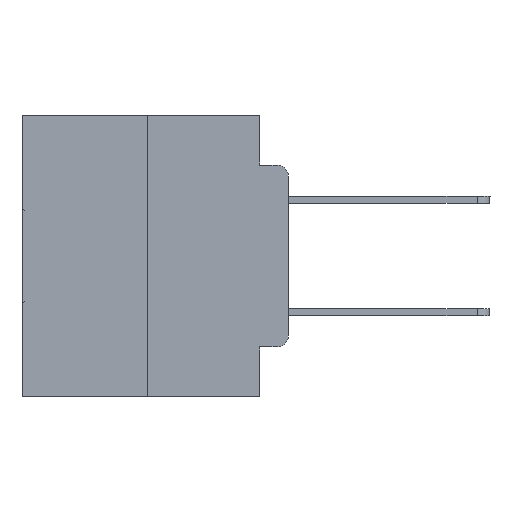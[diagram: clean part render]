
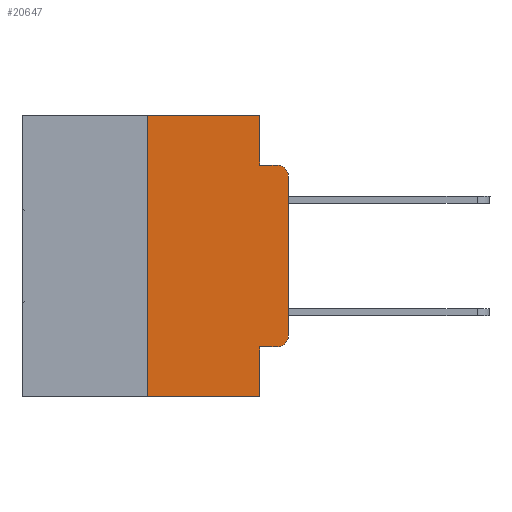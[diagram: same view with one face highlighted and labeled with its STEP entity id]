
A CAD part, left-side view. The second image highlights one B-rep face of the part: STEP entity #20647.
In plain terms, the highlighted planar face has unit normal (-1, 0, 0).
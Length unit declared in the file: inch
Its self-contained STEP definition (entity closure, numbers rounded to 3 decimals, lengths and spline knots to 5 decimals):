
#346 = CARTESIAN_POINT ( 'NONE',  ( 0., 0.051, 0. ) ) ;
#371 = DIRECTION ( 'NONE',  ( 0., 0., -1. ) ) ;
#406 = EDGE_CURVE ( 'NONE', #13097, #30478, #20807, .T. ) ;
#618 = VERTEX_POINT ( 'NONE', #19233 ) ;
#1803 = VERTEX_POINT ( 'NONE', #17296 ) ;
#1904 = EDGE_LOOP ( 'NONE', ( #2455, #10410, #29172, #29894, #11899, #6253, #25933, #15643, #28065, #16396 ) ) ;
#2161 = EDGE_CURVE ( 'NONE', #28129, #618, #17019, .T. ) ;
#2455 = ORIENTED_EDGE ( 'NONE', *, *, #9675, .T. ) ;
#3018 = FACE_OUTER_BOUND ( 'NONE', #1904, .T. ) ;
#3943 = LINE ( 'NONE', #21000, #8900 ) ;
#4062 = LINE ( 'NONE', #24683, #11263 ) ;
#4309 = VECTOR ( 'NONE', #19586, 39.37008 ) ;
#5219 = LINE ( 'NONE', #12419, #10873 ) ;
#5412 = EDGE_CURVE ( 'NONE', #27784, #13097, #4062, .T. ) ;
#5867 = DIRECTION ( 'NONE',  ( 1., 0., 0. ) ) ;
#6253 = ORIENTED_EDGE ( 'NONE', *, *, #5412, .F. ) ;
#6920 = DIRECTION ( 'NONE',  ( -1., 0., 0. ) ) ;
#7275 = EDGE_CURVE ( 'NONE', #27784, #618, #8908, .T. ) ;
#7495 = DIRECTION ( 'NONE',  ( 0., -1., 0. ) ) ;
#7608 = LINE ( 'NONE', #24013, #13200 ) ;
#8628 = DIRECTION ( 'NONE',  ( 0., -1., 0. ) ) ;
#8900 = VECTOR ( 'NONE', #16206, 39.37008 ) ;
#8908 = LINE ( 'NONE', #25203, #15261 ) ;
#9096 = VERTEX_POINT ( 'NONE', #24602 ) ;
#9675 = EDGE_CURVE ( 'NONE', #12359, #27761, #10745, .T. ) ;
#10410 = ORIENTED_EDGE ( 'NONE', *, *, #27595, .T. ) ;
#10500 = DIRECTION ( 'NONE',  ( 0., 0., 1. ) ) ;
#10649 = VECTOR ( 'NONE', #14969, 39.37008 ) ;
#10745 = LINE ( 'NONE', #26467, #4309 ) ;
#10873 = VECTOR ( 'NONE', #371, 39.37008 ) ;
#11010 = DIRECTION ( 'NONE',  ( 0., -1., 0. ) ) ;
#11263 = VECTOR ( 'NONE', #10500, 39.37008 ) ;
#11899 = ORIENTED_EDGE ( 'NONE', *, *, #406, .F. ) ;
#11920 = CARTESIAN_POINT ( 'NONE',  ( 0., 0.051, 0. ) ) ;
#12359 = VERTEX_POINT ( 'NONE', #17969 ) ;
#12419 = CARTESIAN_POINT ( 'NONE',  ( 0., 0.051, 0. ) ) ;
#13097 = VERTEX_POINT ( 'NONE', #29929 ) ;
#13200 = VECTOR ( 'NONE', #7495, 39.37008 ) ;
#14200 = DIRECTION ( 'NONE',  ( -1., 0., 0. ) ) ;
#14438 = VECTOR ( 'NONE', #11010, 39.37008 ) ;
#14717 = AXIS2_PLACEMENT_3D ( 'NONE', #28222, #14200, #30557 ) ;
#14969 = DIRECTION ( 'NONE',  ( 0., 0., -1. ) ) ;
#15261 = VECTOR ( 'NONE', #8628, 39.37008 ) ;
#15643 = ORIENTED_EDGE ( 'NONE', *, *, #2161, .F. ) ;
#16206 = DIRECTION ( 'NONE',  ( 0., -1., 0. ) ) ;
#16396 = ORIENTED_EDGE ( 'NONE', *, *, #21624, .T. ) ;
#17019 = LINE ( 'NONE', #346, #10649 ) ;
#17191 = CARTESIAN_POINT ( 'NONE',  ( 0., 0., -0.1085 ) ) ;
#17296 = CARTESIAN_POINT ( 'NONE',  ( 0., 0.051, -0.0885 ) ) ;
#17969 = CARTESIAN_POINT ( 'NONE',  ( 0., 0., -0.3915 ) ) ;
#19233 = CARTESIAN_POINT ( 'NONE',  ( 0., 0.051, -0.5 ) ) ;
#19586 = DIRECTION ( 'NONE',  ( 0., 0., 1. ) ) ;
#20225 = CARTESIAN_POINT ( 'NONE',  ( 0., 0.473, 0. ) ) ;
#20647 = ADVANCED_FACE ( 'NONE', ( #3018 ), #29409, .F. ) ;
#20807 = LINE ( 'NONE', #21641, #14438 ) ;
#21000 = CARTESIAN_POINT ( 'NONE',  ( 0., 0.051, -0.0885 ) ) ;
#21248 = CARTESIAN_POINT ( 'NONE',  ( 0., 0.02, -0.1085 ) ) ;
#21624 = EDGE_CURVE ( 'NONE', #25698, #12359, #27619, .T. ) ;
#21641 = CARTESIAN_POINT ( 'NONE',  ( 0., 0.473, 0. ) ) ;
#22591 = DIRECTION ( 'NONE',  ( 0., 0., -1. ) ) ;
#22878 = AXIS2_PLACEMENT_3D ( 'NONE', #20225, #5867, #22591 ) ;
#23180 = EDGE_CURVE ( 'NONE', #28129, #25698, #7608, .T. ) ;
#23245 = CARTESIAN_POINT ( 'NONE',  ( 0., 0.051, -0.4115 ) ) ;
#23596 = DIRECTION ( 'NONE',  ( 0., 0., -1. ) ) ;
#24013 = CARTESIAN_POINT ( 'NONE',  ( 0., 0.051, -0.4115 ) ) ;
#24565 = EDGE_CURVE ( 'NONE', #30478, #1803, #5219, .T. ) ;
#24602 = CARTESIAN_POINT ( 'NONE',  ( 0., 0.02, -0.0885 ) ) ;
#24683 = CARTESIAN_POINT ( 'NONE',  ( 0., 0.25, 0. ) ) ;
#24967 = CIRCLE ( 'NONE', #25521, 0.02 ) ;
#25203 = CARTESIAN_POINT ( 'NONE',  ( 0., 0.473, -0.5 ) ) ;
#25521 = AXIS2_PLACEMENT_3D ( 'NONE', #21248, #6920, #23596 ) ;
#25698 = VERTEX_POINT ( 'NONE', #26576 ) ;
#25933 = ORIENTED_EDGE ( 'NONE', *, *, #7275, .T. ) ;
#26091 = EDGE_CURVE ( 'NONE', #1803, #9096, #3943, .T. ) ;
#26467 = CARTESIAN_POINT ( 'NONE',  ( 0., 0., 0. ) ) ;
#26576 = CARTESIAN_POINT ( 'NONE',  ( 0., 0.02, -0.4115 ) ) ;
#27595 = EDGE_CURVE ( 'NONE', #27761, #9096, #24967, .T. ) ;
#27619 = CIRCLE ( 'NONE', #14717, 0.02 ) ;
#27761 = VERTEX_POINT ( 'NONE', #17191 ) ;
#27784 = VERTEX_POINT ( 'NONE', #28894 ) ;
#28065 = ORIENTED_EDGE ( 'NONE', *, *, #23180, .T. ) ;
#28129 = VERTEX_POINT ( 'NONE', #23245 ) ;
#28222 = CARTESIAN_POINT ( 'NONE',  ( 0., 0.02, -0.3915 ) ) ;
#28894 = CARTESIAN_POINT ( 'NONE',  ( 0., 0.25, -0.5 ) ) ;
#29172 = ORIENTED_EDGE ( 'NONE', *, *, #26091, .F. ) ;
#29409 = PLANE ( 'NONE',  #22878 ) ;
#29894 = ORIENTED_EDGE ( 'NONE', *, *, #24565, .F. ) ;
#29929 = CARTESIAN_POINT ( 'NONE',  ( 0., 0.25, 0. ) ) ;
#30478 = VERTEX_POINT ( 'NONE', #11920 ) ;
#30557 = DIRECTION ( 'NONE',  ( 0., 0., -1. ) ) ;
